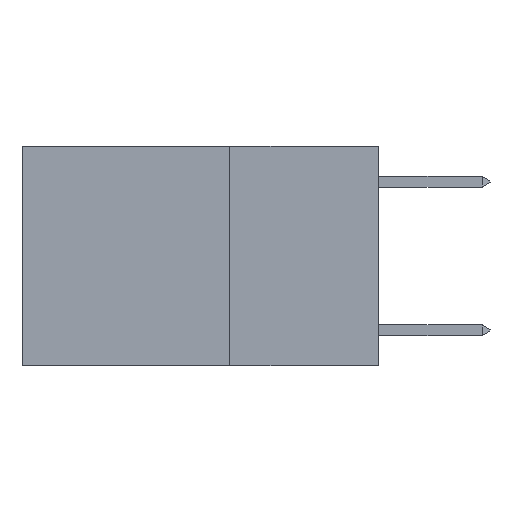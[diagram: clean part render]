
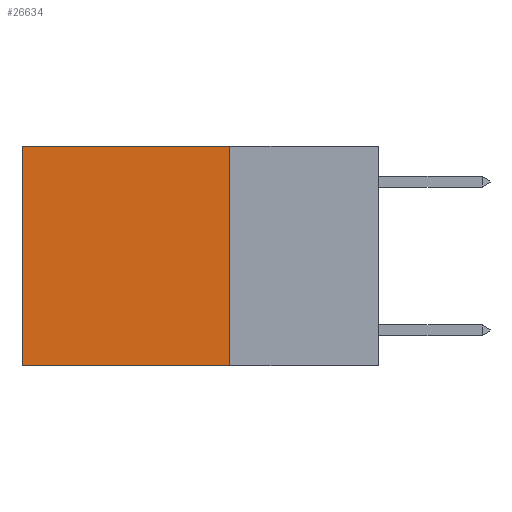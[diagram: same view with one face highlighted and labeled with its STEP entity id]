
A CAD part, left-side view. The second image highlights one B-rep face of the part: STEP entity #26634.
In plain terms, the highlighted planar face has unit normal (-1, 0, 0).
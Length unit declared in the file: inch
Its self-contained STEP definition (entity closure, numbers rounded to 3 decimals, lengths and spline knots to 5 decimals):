
#134 = CARTESIAN_POINT ( 'NONE',  ( 0.2625, 0.6, -0.37 ) ) ;
#272 = VECTOR ( 'NONE', #13543, 39.37008 ) ;
#419 = LINE ( 'NONE', #18031, #272 ) ;
#1796 = LINE ( 'NONE', #3921, #24807 ) ;
#2173 = VERTEX_POINT ( 'NONE', #14537 ) ;
#3921 = CARTESIAN_POINT ( 'NONE',  ( 0.2625, 0.25, -0.37 ) ) ;
#4308 = VECTOR ( 'NONE', #15839, 39.37008 ) ;
#5144 = VERTEX_POINT ( 'NONE', #25092 ) ;
#6854 = ORIENTED_EDGE ( 'NONE', *, *, #11464, .T. ) ;
#6997 = VECTOR ( 'NONE', #14103, 39.37008 ) ;
#7065 = CARTESIAN_POINT ( 'NONE',  ( 0.2625, 0.6, 0. ) ) ;
#7248 = CARTESIAN_POINT ( 'NONE',  ( 0.2625, 0.25, 0. ) ) ;
#7505 = EDGE_LOOP ( 'NONE', ( #6854, #10426, #23725, #26672 ) ) ;
#8754 = PLANE ( 'NONE',  #22851 ) ;
#10426 = ORIENTED_EDGE ( 'NONE', *, *, #14466, .F. ) ;
#10560 = EDGE_CURVE ( 'NONE', #2173, #22178, #27580, .T. ) ;
#11464 = EDGE_CURVE ( 'NONE', #22178, #28077, #17920, .T. ) ;
#13001 = DIRECTION ( 'NONE',  ( 0., 1., 0. ) ) ;
#13543 = DIRECTION ( 'NONE',  ( 0., 0., -1. ) ) ;
#13550 = EDGE_CURVE ( 'NONE', #2173, #5144, #419, .T. ) ;
#13583 = CARTESIAN_POINT ( 'NONE',  ( 0.2625, 0.6, 0. ) ) ;
#14103 = DIRECTION ( 'NONE',  ( 0., 1., 0. ) ) ;
#14466 = EDGE_CURVE ( 'NONE', #5144, #28077, #1796, .T. ) ;
#14537 = CARTESIAN_POINT ( 'NONE',  ( 0.2625, 0.25, 0. ) ) ;
#15037 = DIRECTION ( 'NONE',  ( 0., 0., -1. ) ) ;
#15839 = DIRECTION ( 'NONE',  ( 0., 0., -1. ) ) ;
#17735 = FACE_OUTER_BOUND ( 'NONE', #7505, .T. ) ;
#17858 = CARTESIAN_POINT ( 'NONE',  ( 0.2625, 0.25, 0. ) ) ;
#17920 = LINE ( 'NONE', #13583, #4308 ) ;
#18031 = CARTESIAN_POINT ( 'NONE',  ( 0.2625, 0.25, 0. ) ) ;
#22178 = VERTEX_POINT ( 'NONE', #7065 ) ;
#22851 = AXIS2_PLACEMENT_3D ( 'NONE', #17858, #26999, #15037 ) ;
#23725 = ORIENTED_EDGE ( 'NONE', *, *, #13550, .F. ) ;
#24807 = VECTOR ( 'NONE', #13001, 39.37008 ) ;
#25092 = CARTESIAN_POINT ( 'NONE',  ( 0.2625, 0.25, -0.37 ) ) ;
#26634 = ADVANCED_FACE ( 'NONE', ( #17735 ), #8754, .F. ) ;
#26672 = ORIENTED_EDGE ( 'NONE', *, *, #10560, .T. ) ;
#26999 = DIRECTION ( 'NONE',  ( 1., 0., 0. ) ) ;
#27580 = LINE ( 'NONE', #7248, #6997 ) ;
#28077 = VERTEX_POINT ( 'NONE', #134 ) ;
